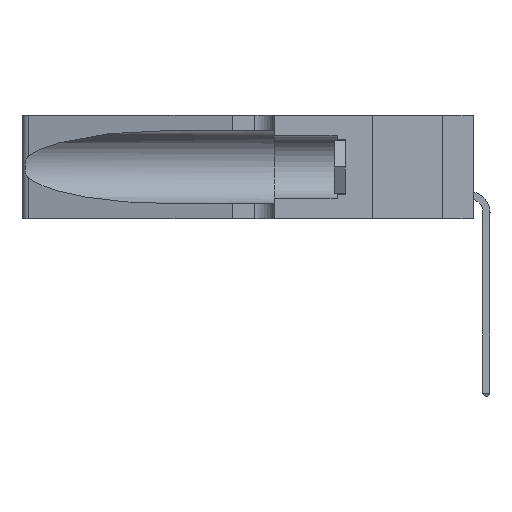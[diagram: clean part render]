
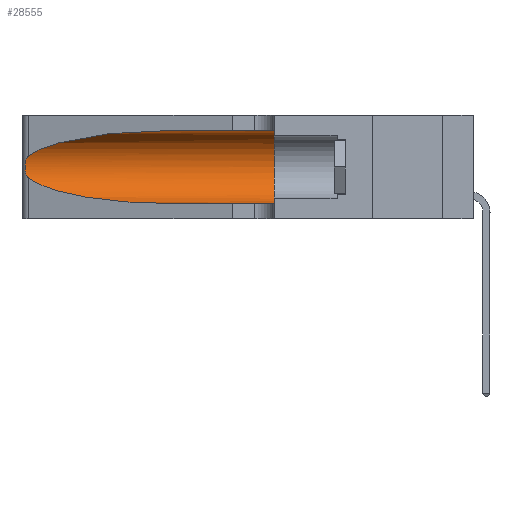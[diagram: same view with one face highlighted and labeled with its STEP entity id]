
A CAD part, left-side view. The second image highlights one B-rep face of the part: STEP entity #28555.
In plain terms, the highlighted cylindrical face has radius 3.308 mm (diameter 6.617 mm), a partial arc.
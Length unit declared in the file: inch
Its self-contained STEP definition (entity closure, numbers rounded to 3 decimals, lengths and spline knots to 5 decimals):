
#921 = EDGE_CURVE ( 'NONE', #1972, #11157, #5606, .T. ) ;
#1426 = CARTESIAN_POINT ( 'NONE',  ( 0.1305, 1.61858, 0.185 ) ) ;
#1972 = VERTEX_POINT ( 'NONE', #19845 ) ;
#2100 = EDGE_CURVE ( 'NONE', #15583, #4080, #22437, .T. ) ;
#2464 = CARTESIAN_POINT ( 'NONE',  ( 0.25487, 1.22718, 0.14631 ) ) ;
#2490 = VECTOR ( 'NONE', #12069, 39.37008 ) ;
#2582 = CARTESIAN_POINT ( 'NONE',  ( 0.1305, 1.61858, 0.05475 ) ) ;
#3208 = CARTESIAN_POINT ( 'NONE',  ( 0.25787, 1.23484, 0.2124 ) ) ;
#3527 = CARTESIAN_POINT ( 'NONE',  ( 0.26075, 1.23896, 0.19203 ) ) ;
#3667 = DIRECTION ( 'NONE',  ( 0., 0., 1. ) ) ;
#4080 = VERTEX_POINT ( 'NONE', #13316 ) ;
#4493 = VERTEX_POINT ( 'NONE', #18384 ) ;
#5606 = LINE ( 'NONE', #24013, #24630 ) ;
#6055 = CARTESIAN_POINT ( 'NONE',  ( 0.25639, 1.23186, 0.15144 ) ) ;
#6088 = CARTESIAN_POINT ( 'NONE',  ( 0.1305, 0.35, 0.185 ) ) ;
#6118 = CARTESIAN_POINT ( 'NONE',  ( 0.25487, 1.22718, 0.22369 ) ) ;
#6219 = CARTESIAN_POINT ( 'NONE',  ( 0.1305, 0.72297, 0.31525 ) ) ;
#6251 = CARTESIAN_POINT ( 'NONE',  ( 0.1305, 0.35, 0.31525 ) ) ;
#7003 = CARTESIAN_POINT ( 'NONE',  ( 0.2373, 1.15595, 0.08982 ) ) ;
#7878 = CYLINDRICAL_SURFACE ( 'NONE', #16195, 0.13025 ) ;
#8143 = CARTESIAN_POINT ( 'NONE',  ( 0.25789, 1.23486, 0.15765 ) ) ;
#9303 = CARTESIAN_POINT ( 'NONE',  ( 0.18966, 0.96281, 0.05475 ) ) ;
#10052 = CARTESIAN_POINT ( 'NONE',  ( 0.25639, 1.23184, 0.21858 ) ) ;
#10558 = CARTESIAN_POINT ( 'NONE',  ( 0.26017, 1.23833, 0.17102 ) ) ;
#11022 = CARTESIAN_POINT ( 'NONE',  ( 0.2373, 1.15595, 0.28018 ) ) ;
#11157 = VERTEX_POINT ( 'NONE', #6251 ) ;
#11527 = LINE ( 'NONE', #2582, #2490 ) ;
#11797 = CIRCLE ( 'NONE', #28582, 0.13025 ) ;
#12069 = DIRECTION ( 'NONE',  ( 0., -1., 0. ) ) ;
#12504 = CARTESIAN_POINT ( 'NONE',  ( 0.26018, 1.23835, 0.19895 ) ) ;
#13316 = CARTESIAN_POINT ( 'NONE',  ( 0.25487, 1.22718, 0.14631 ) ) ;
#13529 = DIRECTION ( 'NONE',  ( 0., -1., 0. ) ) ;
#14734 = FACE_OUTER_BOUND ( 'NONE', #19745, .T. ) ;
#14898 = DIRECTION ( 'NONE',  ( 0., -1., 0. ) ) ;
#15362 = CARTESIAN_POINT ( 'NONE',  ( 0.18966, 0.96281, 0.31525 ) ) ;
#15583 = VERTEX_POINT ( 'NONE', #20988 ) ;
#15678 = CARTESIAN_POINT ( 'NONE',  ( 0.25487, 1.22718, 0.14631 ) ) ;
#15821 =( BOUNDED_CURVE ( )  B_SPLINE_CURVE ( 3, ( #6219, #15362, #11022, #6118 ),
 .UNSPECIFIED., .F., .T. ) 
 B_SPLINE_CURVE_WITH_KNOTS ( ( 4, 4 ),
 ( 1.5708, 2.84003 ),
 .UNSPECIFIED. ) 
 CURVE ( )  GEOMETRIC_REPRESENTATION_ITEM ( )  RATIONAL_B_SPLINE_CURVE ( ( 1., 0.87, 0.87, 1. ) ) 
 REPRESENTATION_ITEM ( '' )  );
#16195 = AXIS2_PLACEMENT_3D ( 'NONE', #1426, #14898, #28703 ) ;
#16721 =( BOUNDED_CURVE ( )  B_SPLINE_CURVE ( 3, ( #2464, #7003, #9303, #25527 ),
 .UNSPECIFIED., .F., .F. ) 
 B_SPLINE_CURVE_WITH_KNOTS ( ( 4, 4 ),
 ( 3.44316, 4.71239 ),
 .UNSPECIFIED. ) 
 CURVE ( )  GEOMETRIC_REPRESENTATION_ITEM ( )  RATIONAL_B_SPLINE_CURVE ( ( 1., 0.87, 0.87, 1. ) ) 
 REPRESENTATION_ITEM ( '' )  );
#18384 = CARTESIAN_POINT ( 'NONE',  ( 0.1305, 0.72297, 0.05475 ) ) ;
#18965 = ORIENTED_EDGE ( 'NONE', *, *, #921, .F. ) ;
#19707 = CARTESIAN_POINT ( 'NONE',  ( 0.25856, 1.23593, 0.16098 ) ) ;
#19745 = EDGE_LOOP ( 'NONE', ( #25048, #26256, #27164, #20310, #20364, #18965 ) ) ;
#19845 = CARTESIAN_POINT ( 'NONE',  ( 0.1305, 0.72297, 0.31525 ) ) ;
#20310 = ORIENTED_EDGE ( 'NONE', *, *, #24321, .T. ) ;
#20364 = ORIENTED_EDGE ( 'NONE', *, *, #20376, .F. ) ;
#20376 = EDGE_CURVE ( 'NONE', #11157, #22689, #11797, .T. ) ;
#20988 = CARTESIAN_POINT ( 'NONE',  ( 0.25487, 1.22718, 0.22369 ) ) ;
#21773 = CARTESIAN_POINT ( 'NONE',  ( 0.26075, 1.23896, 0.178 ) ) ;
#22437 = B_SPLINE_CURVE_WITH_KNOTS ( 'NONE', 3,
 ( #28188, #23670, #10052, #3208, #26169, #12504, #3527, #21773, #10558, #19707, #8143, #6055, #28995, #15678 ),
 .UNSPECIFIED., .F., .F.,
 ( 4, 2, 2, 2, 2, 2, 4 ),
 ( 0., 0.00027, 0.00053, 0.00107, 0.0016, 0.00187, 0.00214 ),
 .UNSPECIFIED. ) ;
#22689 = VERTEX_POINT ( 'NONE', #27788 ) ;
#23670 = CARTESIAN_POINT ( 'NONE',  ( 0.25555, 1.22994, 0.2215 ) ) ;
#24013 = CARTESIAN_POINT ( 'NONE',  ( 0.1305, 1.61858, 0.31525 ) ) ;
#24321 = EDGE_CURVE ( 'NONE', #4493, #22689, #11527, .T. ) ;
#24630 = VECTOR ( 'NONE', #13529, 39.37008 ) ;
#25048 = ORIENTED_EDGE ( 'NONE', *, *, #29430, .T. ) ;
#25420 = EDGE_CURVE ( 'NONE', #4080, #4493, #16721, .T. ) ;
#25527 = CARTESIAN_POINT ( 'NONE',  ( 0.1305, 0.72297, 0.05475 ) ) ;
#26169 = CARTESIAN_POINT ( 'NONE',  ( 0.25854, 1.2359, 0.20912 ) ) ;
#26256 = ORIENTED_EDGE ( 'NONE', *, *, #2100, .T. ) ;
#27164 = ORIENTED_EDGE ( 'NONE', *, *, #25420, .T. ) ;
#27788 = CARTESIAN_POINT ( 'NONE',  ( 0.1305, 0.35, 0.05475 ) ) ;
#28188 = CARTESIAN_POINT ( 'NONE',  ( 0.25487, 1.22718, 0.22369 ) ) ;
#28555 = ADVANCED_FACE ( 'NONE', ( #14734 ), #7878, .F. ) ;
#28582 = AXIS2_PLACEMENT_3D ( 'NONE', #6088, #28736, #3667 ) ;
#28703 = DIRECTION ( 'NONE',  ( 0., 0., -1. ) ) ;
#28736 = DIRECTION ( 'NONE',  ( 0., 1., 0. ) ) ;
#28995 = CARTESIAN_POINT ( 'NONE',  ( 0.25555, 1.22993, 0.14849 ) ) ;
#29430 = EDGE_CURVE ( 'NONE', #1972, #15583, #15821, .T. ) ;
